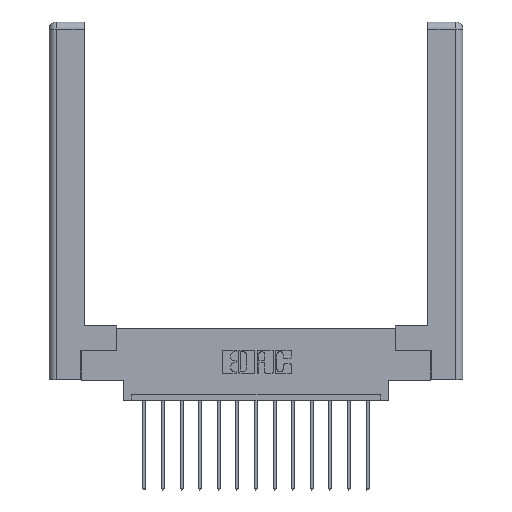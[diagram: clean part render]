
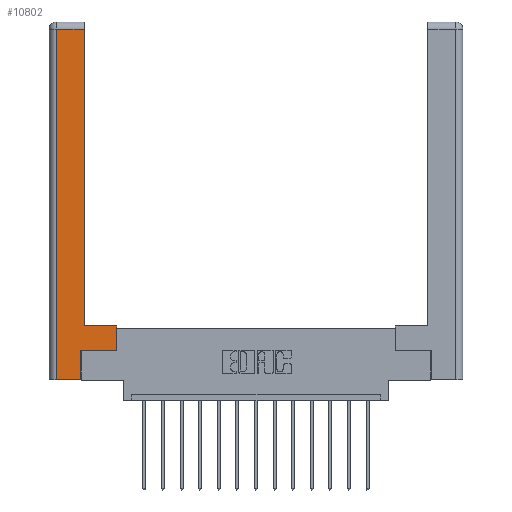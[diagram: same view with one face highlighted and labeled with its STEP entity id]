
A CAD part, top view. The second image highlights one B-rep face of the part: STEP entity #10802.
In plain terms, the highlighted planar face has unit normal (0, 0, 1).
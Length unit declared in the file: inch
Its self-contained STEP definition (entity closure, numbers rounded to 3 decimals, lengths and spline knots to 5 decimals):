
#127 = CARTESIAN_POINT ( 'NONE',  ( 0.0615, 0., 0. ) ) ;
#193 = CARTESIAN_POINT ( 'NONE',  ( 0.565, 0.245, 0. ) ) ;
#222 = CARTESIAN_POINT ( 'NONE',  ( 0.295, 3., 0. ) ) ;
#274 = CARTESIAN_POINT ( 'NONE',  ( 0.565, 0.245, 0. ) ) ;
#566 = CARTESIAN_POINT ( 'NONE',  ( 0.265, 0.245, 0. ) ) ;
#633 = EDGE_LOOP ( 'NONE', ( #13008, #4703, #16196, #7194, #11896, #12642, #9659, #4214 ) ) ;
#1161 = EDGE_CURVE ( 'NONE', #6561, #6296, #8013, .T. ) ;
#1355 = DIRECTION ( 'NONE',  ( 0., 1., 0. ) ) ;
#1626 = LINE ( 'NONE', #14980, #14544 ) ;
#2059 = CARTESIAN_POINT ( 'NONE',  ( 0.265, 0., 0. ) ) ;
#4045 = VECTOR ( 'NONE', #13994, 39.37008 ) ;
#4214 = ORIENTED_EDGE ( 'NONE', *, *, #14622, .T. ) ;
#4228 = VERTEX_POINT ( 'NONE', #127 ) ;
#4447 = VERTEX_POINT ( 'NONE', #8557 ) ;
#4490 = EDGE_CURVE ( 'NONE', #6296, #15116, #4838, .T. ) ;
#4546 = AXIS2_PLACEMENT_3D ( 'NONE', #14467, #4662, #8326 ) ;
#4596 = LINE ( 'NONE', #8510, #15573 ) ;
#4635 = VECTOR ( 'NONE', #15944, 39.37008 ) ;
#4662 = DIRECTION ( 'NONE',  ( 0., 0., -1. ) ) ;
#4703 = ORIENTED_EDGE ( 'NONE', *, *, #13205, .T. ) ;
#4838 = LINE ( 'NONE', #8837, #4045 ) ;
#5027 = VECTOR ( 'NONE', #8273, 39.37008 ) ;
#5843 = VECTOR ( 'NONE', #10501, 39.37008 ) ;
#6219 = LINE ( 'NONE', #2059, #4635 ) ;
#6296 = VERTEX_POINT ( 'NONE', #193 ) ;
#6561 = VERTEX_POINT ( 'NONE', #566 ) ;
#7194 = ORIENTED_EDGE ( 'NONE', *, *, #15194, .T. ) ;
#7444 = CARTESIAN_POINT ( 'NONE',  ( 0.0615, 2.94, 0. ) ) ;
#7480 = DIRECTION ( 'NONE',  ( 0., -1., 0. ) ) ;
#8013 = LINE ( 'NONE', #274, #5843 ) ;
#8094 = VERTEX_POINT ( 'NONE', #15121 ) ;
#8273 = DIRECTION ( 'NONE',  ( -1., 0., 0. ) ) ;
#8326 = DIRECTION ( 'NONE',  ( -1., 0., 0. ) ) ;
#8510 = CARTESIAN_POINT ( 'NONE',  ( 0.265, 0.245, 0. ) ) ;
#8557 = CARTESIAN_POINT ( 'NONE',  ( 0.0615, 2.94, 0. ) ) ;
#8780 = VERTEX_POINT ( 'NONE', #9615 ) ;
#8802 = VERTEX_POINT ( 'NONE', #9105 ) ;
#8837 = CARTESIAN_POINT ( 'NONE',  ( 0.565, 0.45, 0. ) ) ;
#9105 = CARTESIAN_POINT ( 'NONE',  ( 0.295, 2.94, 0. ) ) ;
#9298 = FACE_OUTER_BOUND ( 'NONE', #633, .T. ) ;
#9395 = EDGE_CURVE ( 'NONE', #8780, #8802, #14296, .T. ) ;
#9615 = CARTESIAN_POINT ( 'NONE',  ( 0.295, 0.45, 0. ) ) ;
#9659 = ORIENTED_EDGE ( 'NONE', *, *, #4490, .T. ) ;
#10501 = DIRECTION ( 'NONE',  ( 1., 0., 0. ) ) ;
#10548 = EDGE_CURVE ( 'NONE', #8094, #6561, #4596, .T. ) ;
#10752 = LINE ( 'NONE', #7444, #11510 ) ;
#10802 = ADVANCED_FACE ( 'NONE', ( #9298 ), #13190, .F. ) ;
#11510 = VECTOR ( 'NONE', #16208, 39.37008 ) ;
#11814 = CARTESIAN_POINT ( 'NONE',  ( 0.295, 0.45, 0. ) ) ;
#11841 = EDGE_CURVE ( 'NONE', #4447, #4228, #1626, .T. ) ;
#11896 = ORIENTED_EDGE ( 'NONE', *, *, #10548, .T. ) ;
#12311 = DIRECTION ( 'NONE',  ( 0., 1., 0. ) ) ;
#12642 = ORIENTED_EDGE ( 'NONE', *, *, #1161, .T. ) ;
#13008 = ORIENTED_EDGE ( 'NONE', *, *, #9395, .T. ) ;
#13091 = CARTESIAN_POINT ( 'NONE',  ( 0.565, 0.45, 0. ) ) ;
#13098 = VECTOR ( 'NONE', #1355, 39.37008 ) ;
#13190 = PLANE ( 'NONE',  #4546 ) ;
#13205 = EDGE_CURVE ( 'NONE', #8802, #4447, #10752, .T. ) ;
#13994 = DIRECTION ( 'NONE',  ( 0., 1., 0. ) ) ;
#14296 = LINE ( 'NONE', #222, #13098 ) ;
#14467 = CARTESIAN_POINT ( 'NONE',  ( 0., 0., 0. ) ) ;
#14544 = VECTOR ( 'NONE', #7480, 39.37008 ) ;
#14609 = LINE ( 'NONE', #11814, #5027 ) ;
#14622 = EDGE_CURVE ( 'NONE', #15116, #8780, #14609, .T. ) ;
#14980 = CARTESIAN_POINT ( 'NONE',  ( 0.0615, 0., 0. ) ) ;
#15116 = VERTEX_POINT ( 'NONE', #13091 ) ;
#15121 = CARTESIAN_POINT ( 'NONE',  ( 0.265, 0., 0. ) ) ;
#15194 = EDGE_CURVE ( 'NONE', #4228, #8094, #6219, .T. ) ;
#15573 = VECTOR ( 'NONE', #12311, 39.37008 ) ;
#15944 = DIRECTION ( 'NONE',  ( 1., 0., 0. ) ) ;
#16196 = ORIENTED_EDGE ( 'NONE', *, *, #11841, .T. ) ;
#16208 = DIRECTION ( 'NONE',  ( -1., 0., 0. ) ) ;
